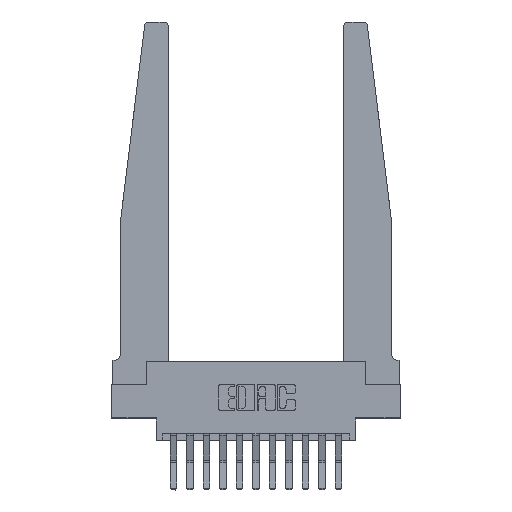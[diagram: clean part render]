
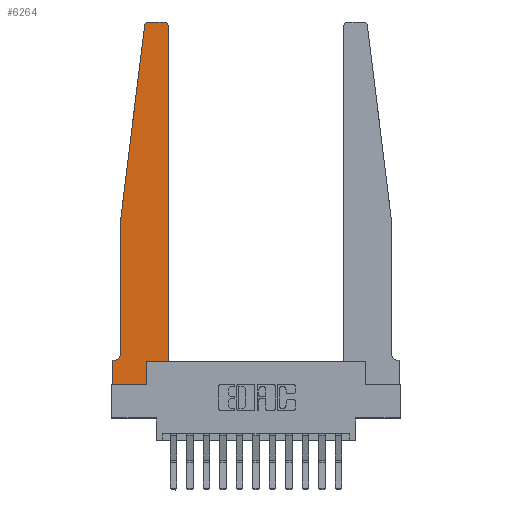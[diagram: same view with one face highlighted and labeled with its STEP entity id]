
A CAD part, top view. The second image highlights one B-rep face of the part: STEP entity #6264.
In plain terms, the highlighted planar face has unit normal (0, 0, 1).
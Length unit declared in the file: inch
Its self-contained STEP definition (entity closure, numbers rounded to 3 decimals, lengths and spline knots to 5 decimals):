
#12 = CARTESIAN_POINT ( 'NONE',  ( 0.2605, 0.18, 0.37 ) ) ;
#56 = DIRECTION ( 'NONE',  ( 1., 0., 0. ) ) ;
#226 = EDGE_CURVE ( 'NONE', #6609, #7321, #3379, .T. ) ;
#244 = EDGE_CURVE ( 'NONE', #7321, #1141, #9200, .T. ) ;
#393 = LINE ( 'NONE', #12605, #6601 ) ;
#409 = CARTESIAN_POINT ( 'NONE',  ( 0.27653, 2.75, 0.37 ) ) ;
#777 = EDGE_CURVE ( 'NONE', #1696, #12190, #12217, .T. ) ;
#967 = VECTOR ( 'NONE', #9824, 39.37008 ) ;
#1141 = VERTEX_POINT ( 'NONE', #409 ) ;
#1186 = DIRECTION ( 'NONE',  ( 0., 0., 1. ) ) ;
#1696 = VERTEX_POINT ( 'NONE', #7445 ) ;
#1885 = VERTEX_POINT ( 'NONE', #14362 ) ;
#2221 = EDGE_CURVE ( 'NONE', #1141, #16310, #7971, .T. ) ;
#2290 = CARTESIAN_POINT ( 'NONE',  ( 0., 0., 0.37 ) ) ;
#2374 = CARTESIAN_POINT ( 'NONE',  ( 0., 0.1875, 0.37 ) ) ;
#2596 = CARTESIAN_POINT ( 'NONE',  ( 0.065, 0.2375, 0.37 ) ) ;
#2632 = LINE ( 'NONE', #2290, #8829 ) ;
#2697 = EDGE_CURVE ( 'NONE', #7109, #13285, #8759, .T. ) ;
#2740 = EDGE_CURVE ( 'NONE', #7932, #1885, #11791, .T. ) ;
#2766 = EDGE_CURVE ( 'NONE', #16310, #1696, #7566, .T. ) ;
#3078 = ORIENTED_EDGE ( 'NONE', *, *, #2221, .T. ) ;
#3379 = CIRCLE ( 'NONE', #13904, 0.03 ) ;
#3396 = EDGE_CURVE ( 'NONE', #1885, #6609, #393, .T. ) ;
#3447 = EDGE_CURVE ( 'NONE', #10184, #12061, #12594, .T. ) ;
#3481 = DIRECTION ( 'NONE',  ( 1., 0., 0. ) ) ;
#3854 = ORIENTED_EDGE ( 'NONE', *, *, #2766, .T. ) ;
#3886 = DIRECTION ( 'NONE',  ( -1., 0., 0. ) ) ;
#4039 = ORIENTED_EDGE ( 'NONE', *, *, #244, .T. ) ;
#4156 = CARTESIAN_POINT ( 'NONE',  ( 0., 0., 0.37 ) ) ;
#4274 = VECTOR ( 'NONE', #16198, 39.37008 ) ;
#4426 = ORIENTED_EDGE ( 'NONE', *, *, #777, .T. ) ;
#4443 = ORIENTED_EDGE ( 'NONE', *, *, #2740, .T. ) ;
#4729 = CIRCLE ( 'NONE', #14752, 0.05 ) ;
#4787 = ORIENTED_EDGE ( 'NONE', *, *, #226, .T. ) ;
#4820 = DIRECTION ( 'NONE',  ( 0., 0., 1. ) ) ;
#5574 = CARTESIAN_POINT ( 'NONE',  ( 0.395, 2.72, 0.37 ) ) ;
#5870 = VECTOR ( 'NONE', #15875, 39.37008 ) ;
#6009 = CARTESIAN_POINT ( 'NONE',  ( 0.425, 0.18, 0.37 ) ) ;
#6070 = LINE ( 'NONE', #12, #9010 ) ;
#6131 = CARTESIAN_POINT ( 'NONE',  ( 0., 0.1875, 0.37 ) ) ;
#6204 = DIRECTION ( 'NONE',  ( 0., 0., -1. ) ) ;
#6264 = ADVANCED_FACE ( 'NONE', ( #9893 ), #8629, .T. ) ;
#6571 = ORIENTED_EDGE ( 'NONE', *, *, #2697, .T. ) ;
#6601 = VECTOR ( 'NONE', #11324, 39.37008 ) ;
#6609 = VERTEX_POINT ( 'NONE', #14437 ) ;
#7109 = VERTEX_POINT ( 'NONE', #4156 ) ;
#7321 = VERTEX_POINT ( 'NONE', #13187 ) ;
#7445 = CARTESIAN_POINT ( 'NONE',  ( 0.065, 1.25, 0.37 ) ) ;
#7489 = DIRECTION ( 'NONE',  ( 0., 0., 1. ) ) ;
#7541 = EDGE_CURVE ( 'NONE', #12061, #7109, #2632, .T. ) ;
#7566 = LINE ( 'NONE', #8511, #967 ) ;
#7932 = VERTEX_POINT ( 'NONE', #15836 ) ;
#7971 = CIRCLE ( 'NONE', #15327, 0.03 ) ;
#8250 = EDGE_CURVE ( 'NONE', #13285, #7932, #6070, .T. ) ;
#8356 = VECTOR ( 'NONE', #3481, 39.37008 ) ;
#8511 = CARTESIAN_POINT ( 'NONE',  ( 0.065, 1.25, 0.37 ) ) ;
#8629 = PLANE ( 'NONE',  #15478 ) ;
#8759 = LINE ( 'NONE', #11011, #8356 ) ;
#8765 = EDGE_LOOP ( 'NONE', ( #4039, #3078, #3854, #4426, #10955, #14729, #15135, #6571, #10353, #4443, #11992, #4787 ) ) ;
#8829 = VECTOR ( 'NONE', #14782, 39.37008 ) ;
#9010 = VECTOR ( 'NONE', #10027, 39.37008 ) ;
#9200 = LINE ( 'NONE', #10204, #5870 ) ;
#9824 = DIRECTION ( 'NONE',  ( -0.122, -0.992, 0. ) ) ;
#9893 = FACE_OUTER_BOUND ( 'NONE', #8765, .T. ) ;
#9944 = DIRECTION ( 'NONE',  ( 1., 0., 0. ) ) ;
#9975 = CARTESIAN_POINT ( 'NONE',  ( 0.24675, 2.72367, 0.37 ) ) ;
#10027 = DIRECTION ( 'NONE',  ( 0., 1., 0. ) ) ;
#10184 = VERTEX_POINT ( 'NONE', #14318 ) ;
#10204 = CARTESIAN_POINT ( 'NONE',  ( 0.25, 2.75, 0.37 ) ) ;
#10353 = ORIENTED_EDGE ( 'NONE', *, *, #8250, .T. ) ;
#10443 = EDGE_CURVE ( 'NONE', #12190, #10184, #4729, .T. ) ;
#10955 = ORIENTED_EDGE ( 'NONE', *, *, #10443, .T. ) ;
#11011 = CARTESIAN_POINT ( 'NONE',  ( 0., 0., 0.37 ) ) ;
#11324 = DIRECTION ( 'NONE',  ( 0., 1., 0. ) ) ;
#11429 = VECTOR ( 'NONE', #12974, 39.37008 ) ;
#11791 = LINE ( 'NONE', #6009, #4274 ) ;
#11992 = ORIENTED_EDGE ( 'NONE', *, *, #3396, .T. ) ;
#12061 = VERTEX_POINT ( 'NONE', #2374 ) ;
#12190 = VERTEX_POINT ( 'NONE', #2596 ) ;
#12217 = LINE ( 'NONE', #13008, #11429 ) ;
#12517 = CARTESIAN_POINT ( 'NONE',  ( 0.2605, 0., 0.37 ) ) ;
#12594 = LINE ( 'NONE', #12715, #15972 ) ;
#12605 = CARTESIAN_POINT ( 'NONE',  ( 0.425, 0.18, 0.37 ) ) ;
#12715 = CARTESIAN_POINT ( 'NONE',  ( 0.065, 0.1875, 0.37 ) ) ;
#12974 = DIRECTION ( 'NONE',  ( 0., -1., 0. ) ) ;
#13008 = CARTESIAN_POINT ( 'NONE',  ( 0.065, 1.25, 0.37 ) ) ;
#13187 = CARTESIAN_POINT ( 'NONE',  ( 0.395, 2.75, 0.37 ) ) ;
#13285 = VERTEX_POINT ( 'NONE', #12517 ) ;
#13823 = CARTESIAN_POINT ( 'NONE',  ( 0.015, 0.2375, 0.37 ) ) ;
#13904 = AXIS2_PLACEMENT_3D ( 'NONE', #5574, #4820, #14845 ) ;
#14318 = CARTESIAN_POINT ( 'NONE',  ( 0.015, 0.1875, 0.37 ) ) ;
#14362 = CARTESIAN_POINT ( 'NONE',  ( 0.425, 0.18, 0.37 ) ) ;
#14437 = CARTESIAN_POINT ( 'NONE',  ( 0.425, 2.72, 0.37 ) ) ;
#14729 = ORIENTED_EDGE ( 'NONE', *, *, #3447, .T. ) ;
#14752 = AXIS2_PLACEMENT_3D ( 'NONE', #13823, #6204, #15090 ) ;
#14782 = DIRECTION ( 'NONE',  ( 0., -1., 0. ) ) ;
#14845 = DIRECTION ( 'NONE',  ( 1., 0., 0. ) ) ;
#15090 = DIRECTION ( 'NONE',  ( -1., 0., 0. ) ) ;
#15135 = ORIENTED_EDGE ( 'NONE', *, *, #7541, .T. ) ;
#15139 = CARTESIAN_POINT ( 'NONE',  ( 0.27653, 2.72, 0.37 ) ) ;
#15327 = AXIS2_PLACEMENT_3D ( 'NONE', #15139, #7489, #56 ) ;
#15478 = AXIS2_PLACEMENT_3D ( 'NONE', #6131, #1186, #9944 ) ;
#15836 = CARTESIAN_POINT ( 'NONE',  ( 0.2605, 0.18, 0.37 ) ) ;
#15875 = DIRECTION ( 'NONE',  ( -1., 0., 0. ) ) ;
#15972 = VECTOR ( 'NONE', #3886, 39.37008 ) ;
#16198 = DIRECTION ( 'NONE',  ( 1., 0., 0. ) ) ;
#16310 = VERTEX_POINT ( 'NONE', #9975 ) ;
